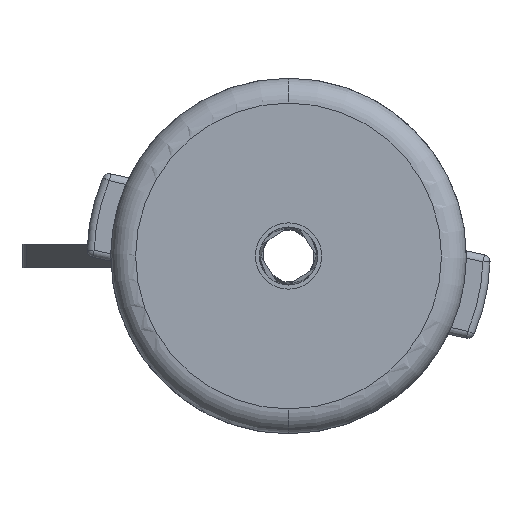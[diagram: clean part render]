
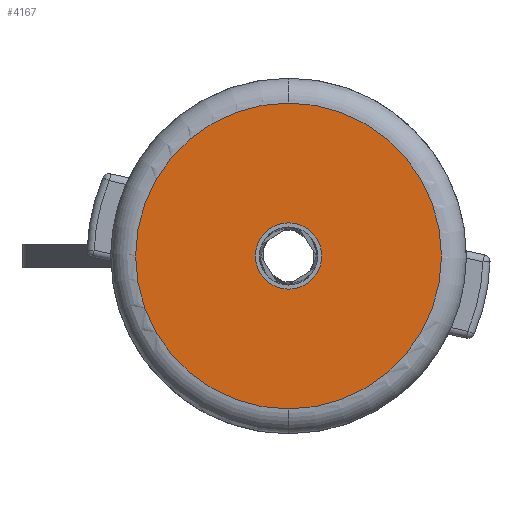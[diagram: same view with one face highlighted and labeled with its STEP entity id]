
A CAD part, front view. The second image highlights one B-rep face of the part: STEP entity #4167.
In plain terms, the highlighted planar face has unit normal (0, -1, 0).
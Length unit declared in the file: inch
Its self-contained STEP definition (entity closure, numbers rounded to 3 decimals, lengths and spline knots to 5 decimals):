
#42 = CIRCLE ( 'NONE', #6203, 0.14 ) ;
#324 = CARTESIAN_POINT ( 'NONE',  ( 0., 0., 0. ) ) ;
#375 = CARTESIAN_POINT ( 'NONE',  ( 0., 0., 0. ) ) ;
#627 = AXIS2_PLACEMENT_3D ( 'NONE', #375, #9829, #1730 ) ;
#1407 = CIRCLE ( 'NONE', #1586, 0.14 ) ;
#1586 = AXIS2_PLACEMENT_3D ( 'NONE', #6483, #15917, #7834 ) ;
#1686 = DIRECTION ( 'NONE',  ( 0., 0., -1. ) ) ;
#1730 = DIRECTION ( 'NONE',  ( 0., 0., -1. ) ) ;
#1900 = CIRCLE ( 'NONE', #627, 0.645 ) ;
#1952 = VERTEX_POINT ( 'NONE', #4527 ) ;
#2068 = EDGE_LOOP ( 'NONE', ( #11240, #10199 ) ) ;
#2137 = EDGE_CURVE ( 'NONE', #1952, #2867, #42, .T. ) ;
#2815 = AXIS2_PLACEMENT_3D ( 'NONE', #6301, #15724, #7649 ) ;
#2867 = VERTEX_POINT ( 'NONE', #12816 ) ;
#3603 = CIRCLE ( 'NONE', #2815, 0.645 ) ;
#4058 = ORIENTED_EDGE ( 'NONE', *, *, #11892, .T. ) ;
#4069 = FACE_OUTER_BOUND ( 'NONE', #2068, .T. ) ;
#4167 = ADVANCED_FACE ( 'NONE', ( #4069, #16095 ), #15170, .T. ) ;
#4527 = CARTESIAN_POINT ( 'NONE',  ( 0., 0., 0.14 ) ) ;
#6118 = EDGE_CURVE ( 'NONE', #16918, #14654, #3603, .T. ) ;
#6203 = AXIS2_PLACEMENT_3D ( 'NONE', #16161, #8083, #17513 ) ;
#6301 = CARTESIAN_POINT ( 'NONE',  ( 0., 0., 0. ) ) ;
#6483 = CARTESIAN_POINT ( 'NONE',  ( 0., 0., 0. ) ) ;
#6910 = EDGE_CURVE ( 'NONE', #14654, #16918, #1900, .T. ) ;
#7649 = DIRECTION ( 'NONE',  ( 0., 0., -1. ) ) ;
#7834 = DIRECTION ( 'NONE',  ( 0., 0., 1. ) ) ;
#8083 = DIRECTION ( 'NONE',  ( 0., 1., 0. ) ) ;
#9282 = ORIENTED_EDGE ( 'NONE', *, *, #2137, .T. ) ;
#9331 = EDGE_LOOP ( 'NONE', ( #4058, #9282 ) ) ;
#9509 = CARTESIAN_POINT ( 'NONE',  ( 0., 0., 0.645 ) ) ;
#9718 = AXIS2_PLACEMENT_3D ( 'NONE', #324, #9785, #1686 ) ;
#9785 = DIRECTION ( 'NONE',  ( 0., -1., 0. ) ) ;
#9829 = DIRECTION ( 'NONE',  ( 0., -1., 0. ) ) ;
#10199 = ORIENTED_EDGE ( 'NONE', *, *, #6118, .T. ) ;
#11240 = ORIENTED_EDGE ( 'NONE', *, *, #6910, .T. ) ;
#11892 = EDGE_CURVE ( 'NONE', #2867, #1952, #1407, .T. ) ;
#12313 = CARTESIAN_POINT ( 'NONE',  ( 0., 0., -0.645 ) ) ;
#12816 = CARTESIAN_POINT ( 'NONE',  ( 0., 0., -0.14 ) ) ;
#14654 = VERTEX_POINT ( 'NONE', #12313 ) ;
#15170 = PLANE ( 'NONE',  #9718 ) ;
#15724 = DIRECTION ( 'NONE',  ( 0., -1., 0. ) ) ;
#15917 = DIRECTION ( 'NONE',  ( 0., 1., 0. ) ) ;
#16095 = FACE_BOUND ( 'NONE', #9331, .T. ) ;
#16161 = CARTESIAN_POINT ( 'NONE',  ( 0., 0., 0. ) ) ;
#16918 = VERTEX_POINT ( 'NONE', #9509 ) ;
#17513 = DIRECTION ( 'NONE',  ( 0., 0., 1. ) ) ;
